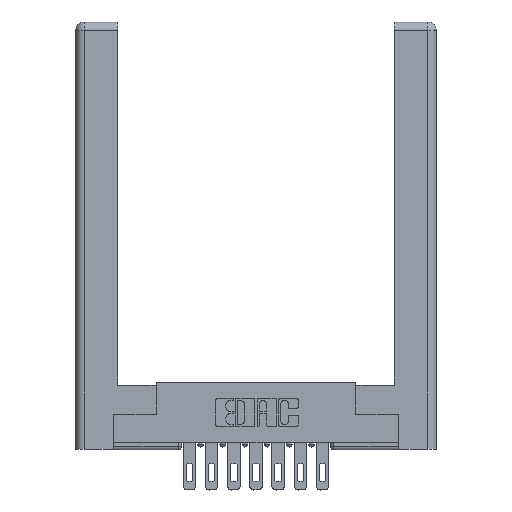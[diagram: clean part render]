
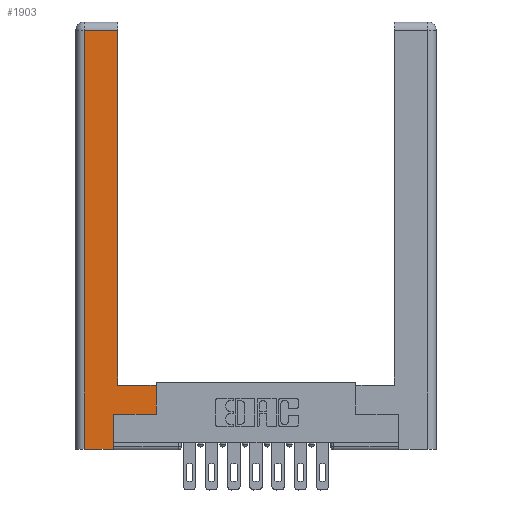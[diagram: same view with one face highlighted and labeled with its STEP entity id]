
A CAD part, top view. The second image highlights one B-rep face of the part: STEP entity #1903.
In plain terms, the highlighted planar face has unit normal (0, 0, 1).
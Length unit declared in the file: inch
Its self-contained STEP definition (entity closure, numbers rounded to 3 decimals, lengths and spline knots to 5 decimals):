
#86 = EDGE_CURVE ( 'NONE', #6829, #9431, #2495, .T. ) ;
#371 = DIRECTION ( 'NONE',  ( -1., 0., 0. ) ) ;
#472 = LINE ( 'NONE', #8286, #2676 ) ;
#492 = PLANE ( 'NONE',  #6748 ) ;
#674 = CARTESIAN_POINT ( 'NONE',  ( 0.565, 0.45, 0. ) ) ;
#1368 = ORIENTED_EDGE ( 'NONE', *, *, #5696, .T. ) ;
#1408 = CARTESIAN_POINT ( 'NONE',  ( 0.265, 0.245, 0. ) ) ;
#1564 = VECTOR ( 'NONE', #7197, 39.37008 ) ;
#1625 = FACE_OUTER_BOUND ( 'NONE', #3617, .T. ) ;
#1903 = ADVANCED_FACE ( 'NONE', ( #1625 ), #492, .F. ) ;
#2023 = LINE ( 'NONE', #5293, #4036 ) ;
#2495 = LINE ( 'NONE', #11638, #11230 ) ;
#2653 = LINE ( 'NONE', #8383, #1564 ) ;
#2676 = VECTOR ( 'NONE', #5249, 39.37008 ) ;
#2701 = ORIENTED_EDGE ( 'NONE', *, *, #7850, .T. ) ;
#3185 = CARTESIAN_POINT ( 'NONE',  ( 0.295, 3., 0. ) ) ;
#3382 = EDGE_CURVE ( 'NONE', #9984, #3714, #3626, .T. ) ;
#3409 = DIRECTION ( 'NONE',  ( 0., 0., -1. ) ) ;
#3617 = EDGE_LOOP ( 'NONE', ( #4515, #3795, #1368, #8532, #3919, #2701, #10506, #3686 ) ) ;
#3626 = LINE ( 'NONE', #11274, #8402 ) ;
#3686 = ORIENTED_EDGE ( 'NONE', *, *, #4925, .T. ) ;
#3714 = VERTEX_POINT ( 'NONE', #7811 ) ;
#3795 = ORIENTED_EDGE ( 'NONE', *, *, #86, .T. ) ;
#3919 = ORIENTED_EDGE ( 'NONE', *, *, #11251, .T. ) ;
#4036 = VECTOR ( 'NONE', #9363, 39.37008 ) ;
#4133 = CARTESIAN_POINT ( 'NONE',  ( 0.295, 2.94, 0. ) ) ;
#4197 = VECTOR ( 'NONE', #10668, 39.37008 ) ;
#4515 = ORIENTED_EDGE ( 'NONE', *, *, #7254, .T. ) ;
#4925 = EDGE_CURVE ( 'NONE', #13135, #11195, #2653, .T. ) ;
#5249 = DIRECTION ( 'NONE',  ( 0., 1., 0. ) ) ;
#5293 = CARTESIAN_POINT ( 'NONE',  ( 0.565, 0.245, 0. ) ) ;
#5417 = LINE ( 'NONE', #1408, #7647 ) ;
#5696 = EDGE_CURVE ( 'NONE', #9431, #9984, #10734, .T. ) ;
#6130 = CARTESIAN_POINT ( 'NONE',  ( 0.0615, 2.94, 0. ) ) ;
#6411 = DIRECTION ( 'NONE',  ( 0., 1., 0. ) ) ;
#6629 = LINE ( 'NONE', #3185, #12069 ) ;
#6748 = AXIS2_PLACEMENT_3D ( 'NONE', #9513, #3409, #12624 ) ;
#6829 = VERTEX_POINT ( 'NONE', #4133 ) ;
#7197 = DIRECTION ( 'NONE',  ( -1., 0., 0. ) ) ;
#7254 = EDGE_CURVE ( 'NONE', #11195, #6829, #6629, .T. ) ;
#7260 = DIRECTION ( 'NONE',  ( 1., 0., 0. ) ) ;
#7604 = CARTESIAN_POINT ( 'NONE',  ( 0.0615, 0., 0. ) ) ;
#7647 = VECTOR ( 'NONE', #6411, 39.37008 ) ;
#7811 = CARTESIAN_POINT ( 'NONE',  ( 0.265, 0., 0. ) ) ;
#7850 = EDGE_CURVE ( 'NONE', #9069, #9042, #2023, .T. ) ;
#8286 = CARTESIAN_POINT ( 'NONE',  ( 0.565, 0.45, 0. ) ) ;
#8383 = CARTESIAN_POINT ( 'NONE',  ( 0.295, 0.45, 0. ) ) ;
#8402 = VECTOR ( 'NONE', #7260, 39.37008 ) ;
#8522 = DIRECTION ( 'NONE',  ( 0., 1., 0. ) ) ;
#8532 = ORIENTED_EDGE ( 'NONE', *, *, #3382, .T. ) ;
#8562 = CARTESIAN_POINT ( 'NONE',  ( 0.565, 0.245, 0. ) ) ;
#9042 = VERTEX_POINT ( 'NONE', #8562 ) ;
#9069 = VERTEX_POINT ( 'NONE', #9549 ) ;
#9363 = DIRECTION ( 'NONE',  ( 1., 0., 0. ) ) ;
#9431 = VERTEX_POINT ( 'NONE', #6130 ) ;
#9513 = CARTESIAN_POINT ( 'NONE',  ( 0., 0., 0. ) ) ;
#9549 = CARTESIAN_POINT ( 'NONE',  ( 0.265, 0.245, 0. ) ) ;
#9936 = CARTESIAN_POINT ( 'NONE',  ( 0.0615, 0., 0. ) ) ;
#9984 = VERTEX_POINT ( 'NONE', #9936 ) ;
#10506 = ORIENTED_EDGE ( 'NONE', *, *, #12796, .T. ) ;
#10668 = DIRECTION ( 'NONE',  ( 0., -1., 0. ) ) ;
#10734 = LINE ( 'NONE', #7604, #4197 ) ;
#11195 = VERTEX_POINT ( 'NONE', #12592 ) ;
#11230 = VECTOR ( 'NONE', #371, 39.37008 ) ;
#11251 = EDGE_CURVE ( 'NONE', #3714, #9069, #5417, .T. ) ;
#11274 = CARTESIAN_POINT ( 'NONE',  ( 0.265, 0., 0. ) ) ;
#11638 = CARTESIAN_POINT ( 'NONE',  ( 0.0615, 2.94, 0. ) ) ;
#12069 = VECTOR ( 'NONE', #8522, 39.37008 ) ;
#12592 = CARTESIAN_POINT ( 'NONE',  ( 0.295, 0.45, 0. ) ) ;
#12624 = DIRECTION ( 'NONE',  ( -1., 0., 0. ) ) ;
#12796 = EDGE_CURVE ( 'NONE', #9042, #13135, #472, .T. ) ;
#13135 = VERTEX_POINT ( 'NONE', #674 ) ;
